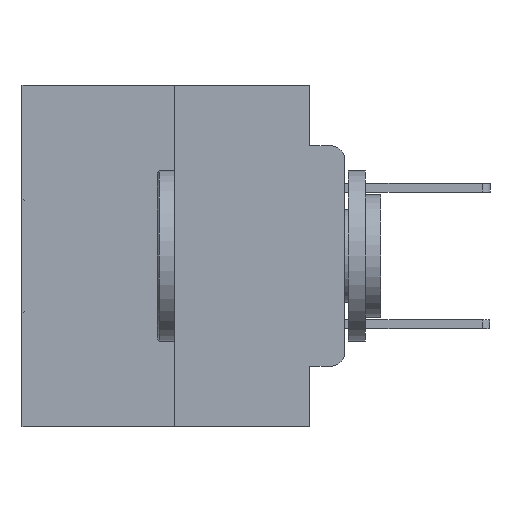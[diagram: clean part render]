
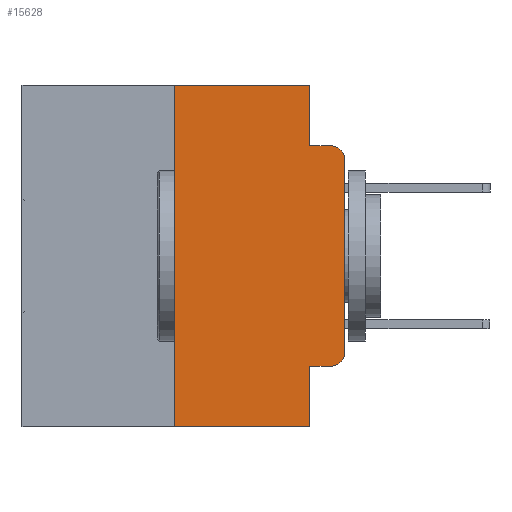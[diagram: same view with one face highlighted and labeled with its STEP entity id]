
A CAD part, left-side view. The second image highlights one B-rep face of the part: STEP entity #15628.
In plain terms, the highlighted planar face has unit normal (-1, 0, 0).
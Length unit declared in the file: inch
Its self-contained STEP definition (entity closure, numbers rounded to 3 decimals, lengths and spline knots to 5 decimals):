
#749 = ORIENTED_EDGE ( 'NONE', *, *, #25771, .T. ) ;
#1101 = VERTEX_POINT ( 'NONE', #21882 ) ;
#1860 = DIRECTION ( 'NONE',  ( 0., 0., 1. ) ) ;
#1887 = ORIENTED_EDGE ( 'NONE', *, *, #3491, .T. ) ;
#2306 = ORIENTED_EDGE ( 'NONE', *, *, #13436, .F. ) ;
#2916 = DIRECTION ( 'NONE',  ( 0., -1., 0. ) ) ;
#2937 = VERTEX_POINT ( 'NONE', #26197 ) ;
#3296 = AXIS2_PLACEMENT_3D ( 'NONE', #3409, #20207, #5887 ) ;
#3409 = CARTESIAN_POINT ( 'NONE',  ( 0., 0.02, -0.3915 ) ) ;
#3469 = ORIENTED_EDGE ( 'NONE', *, *, #28157, .F. ) ;
#3491 = EDGE_CURVE ( 'NONE', #12858, #17508, #29679, .T. ) ;
#3839 = VECTOR ( 'NONE', #22882, 39.37008 ) ;
#4625 = CARTESIAN_POINT ( 'NONE',  ( 0., 0.25, 0. ) ) ;
#5301 = LINE ( 'NONE', #28583, #17298 ) ;
#5550 = PLANE ( 'NONE',  #23970 ) ;
#5809 = VERTEX_POINT ( 'NONE', #6459 ) ;
#5827 = DIRECTION ( 'NONE',  ( 0., 0., -1. ) ) ;
#5887 = DIRECTION ( 'NONE',  ( 0., 0., -1. ) ) ;
#5983 = LINE ( 'NONE', #28141, #24268 ) ;
#6172 = CARTESIAN_POINT ( 'NONE',  ( 0., 0.051, -0.4115 ) ) ;
#6459 = CARTESIAN_POINT ( 'NONE',  ( 0., 0.051, 0. ) ) ;
#6948 = EDGE_CURVE ( 'NONE', #9822, #12858, #29825, .T. ) ;
#8031 = VERTEX_POINT ( 'NONE', #15118 ) ;
#8094 = CARTESIAN_POINT ( 'NONE',  ( 0., 0.051, -0.5 ) ) ;
#8888 = ORIENTED_EDGE ( 'NONE', *, *, #10244, .T. ) ;
#9175 = CARTESIAN_POINT ( 'NONE',  ( 0., 0., -0.1085 ) ) ;
#9822 = VERTEX_POINT ( 'NONE', #16479 ) ;
#9826 = EDGE_LOOP ( 'NONE', ( #1887, #21861, #3469, #29665, #17758, #19253, #749, #2306, #8888, #27813 ) ) ;
#10244 = EDGE_CURVE ( 'NONE', #2937, #9822, #30014, .T. ) ;
#10321 = CARTESIAN_POINT ( 'NONE',  ( 0., 0.473, 0. ) ) ;
#10454 = DIRECTION ( 'NONE',  ( 0., 0., -1. ) ) ;
#11816 = CARTESIAN_POINT ( 'NONE',  ( 0., 0., 0. ) ) ;
#11818 = VECTOR ( 'NONE', #2916, 39.37008 ) ;
#12858 = VERTEX_POINT ( 'NONE', #24241 ) ;
#13436 = EDGE_CURVE ( 'NONE', #2937, #13637, #16454, .T. ) ;
#13637 = VERTEX_POINT ( 'NONE', #8094 ) ;
#13660 = VECTOR ( 'NONE', #5827, 39.37008 ) ;
#13751 = CARTESIAN_POINT ( 'NONE',  ( 0., 0.02, -0.1085 ) ) ;
#14300 = CARTESIAN_POINT ( 'NONE',  ( 0., 0.02, -0.0885 ) ) ;
#15118 = CARTESIAN_POINT ( 'NONE',  ( 0., 0.051, -0.0885 ) ) ;
#15607 = VECTOR ( 'NONE', #21394, 39.37008 ) ;
#15628 = ADVANCED_FACE ( 'NONE', ( #25716 ), #5550, .F. ) ;
#16113 = DIRECTION ( 'NONE',  ( 0., 0., -1. ) ) ;
#16306 = DIRECTION ( 'NONE',  ( 0., -1., 0. ) ) ;
#16454 = LINE ( 'NONE', #23911, #28341 ) ;
#16479 = CARTESIAN_POINT ( 'NONE',  ( 0., 0.02, -0.4115 ) ) ;
#17150 = CIRCLE ( 'NONE', #20467, 0.02 ) ;
#17298 = VECTOR ( 'NONE', #30910, 39.37008 ) ;
#17329 = LINE ( 'NONE', #10321, #11818 ) ;
#17508 = VERTEX_POINT ( 'NONE', #9175 ) ;
#17758 = ORIENTED_EDGE ( 'NONE', *, *, #19630, .F. ) ;
#18156 = EDGE_CURVE ( 'NONE', #19003, #1101, #22629, .T. ) ;
#19003 = VERTEX_POINT ( 'NONE', #19879 ) ;
#19253 = ORIENTED_EDGE ( 'NONE', *, *, #18156, .F. ) ;
#19630 = EDGE_CURVE ( 'NONE', #1101, #5809, #17329, .T. ) ;
#19761 = EDGE_CURVE ( 'NONE', #5809, #8031, #26239, .T. ) ;
#19879 = CARTESIAN_POINT ( 'NONE',  ( 0., 0.25, -0.5 ) ) ;
#20207 = DIRECTION ( 'NONE',  ( -1., 0., 0. ) ) ;
#20467 = AXIS2_PLACEMENT_3D ( 'NONE', #13751, #30296, #16113 ) ;
#21394 = DIRECTION ( 'NONE',  ( 0., 0., 1. ) ) ;
#21861 = ORIENTED_EDGE ( 'NONE', *, *, #29740, .T. ) ;
#21882 = CARTESIAN_POINT ( 'NONE',  ( 0., 0.25, 0. ) ) ;
#22261 = CARTESIAN_POINT ( 'NONE',  ( 0., 0.473, 0. ) ) ;
#22629 = LINE ( 'NONE', #4625, #15607 ) ;
#22882 = DIRECTION ( 'NONE',  ( 0., -1., 0. ) ) ;
#23353 = VECTOR ( 'NONE', #1860, 39.37008 ) ;
#23911 = CARTESIAN_POINT ( 'NONE',  ( 0., 0.051, 0. ) ) ;
#23970 = AXIS2_PLACEMENT_3D ( 'NONE', #22261, #24642, #10454 ) ;
#24241 = CARTESIAN_POINT ( 'NONE',  ( 0., 0., -0.3915 ) ) ;
#24268 = VECTOR ( 'NONE', #16306, 39.37008 ) ;
#24642 = DIRECTION ( 'NONE',  ( 1., 0., 0. ) ) ;
#25422 = VERTEX_POINT ( 'NONE', #14300 ) ;
#25716 = FACE_OUTER_BOUND ( 'NONE', #9826, .T. ) ;
#25771 = EDGE_CURVE ( 'NONE', #19003, #13637, #5301, .T. ) ;
#26197 = CARTESIAN_POINT ( 'NONE',  ( 0., 0.051, -0.4115 ) ) ;
#26239 = LINE ( 'NONE', #29702, #13660 ) ;
#27813 = ORIENTED_EDGE ( 'NONE', *, *, #6948, .T. ) ;
#28141 = CARTESIAN_POINT ( 'NONE',  ( 0., 0.051, -0.0885 ) ) ;
#28157 = EDGE_CURVE ( 'NONE', #8031, #25422, #5983, .T. ) ;
#28341 = VECTOR ( 'NONE', #28706, 39.37008 ) ;
#28583 = CARTESIAN_POINT ( 'NONE',  ( 0., 0.473, -0.5 ) ) ;
#28706 = DIRECTION ( 'NONE',  ( 0., 0., -1. ) ) ;
#29665 = ORIENTED_EDGE ( 'NONE', *, *, #19761, .F. ) ;
#29679 = LINE ( 'NONE', #11816, #23353 ) ;
#29702 = CARTESIAN_POINT ( 'NONE',  ( 0., 0.051, 0. ) ) ;
#29740 = EDGE_CURVE ( 'NONE', #17508, #25422, #17150, .T. ) ;
#29825 = CIRCLE ( 'NONE', #3296, 0.02 ) ;
#30014 = LINE ( 'NONE', #6172, #3839 ) ;
#30296 = DIRECTION ( 'NONE',  ( -1., 0., 0. ) ) ;
#30910 = DIRECTION ( 'NONE',  ( 0., -1., 0. ) ) ;
